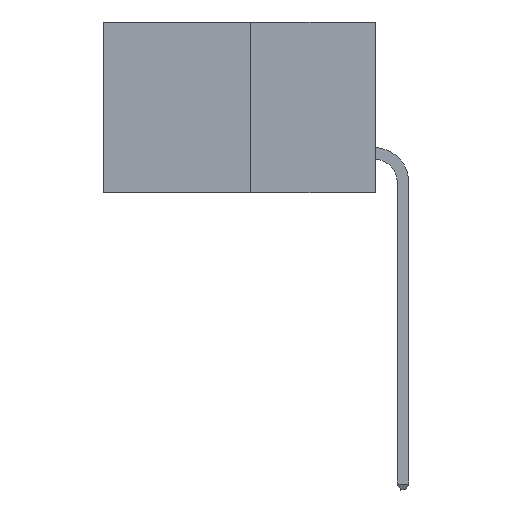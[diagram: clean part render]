
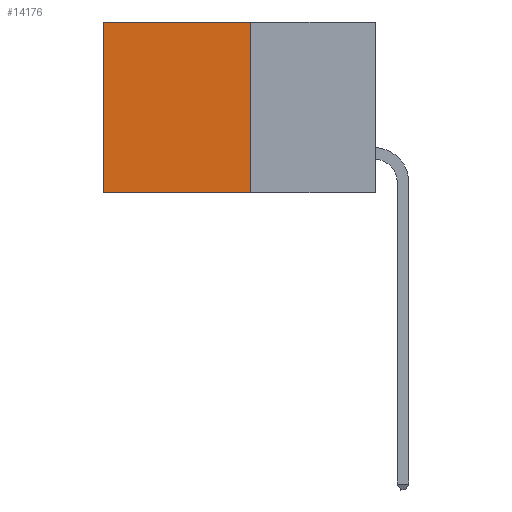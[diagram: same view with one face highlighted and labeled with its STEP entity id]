
A CAD part, left-side view. The second image highlights one B-rep face of the part: STEP entity #14176.
In plain terms, the highlighted planar face has unit normal (-1, 0, 0).
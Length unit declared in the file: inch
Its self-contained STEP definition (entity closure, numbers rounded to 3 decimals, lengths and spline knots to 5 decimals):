
#125 = CARTESIAN_POINT ( 'NONE',  ( 0.277, 0.27, -0.37 ) ) ;
#161 = VERTEX_POINT ( 'NONE', #10917 ) ;
#1393 = CARTESIAN_POINT ( 'NONE',  ( 0.277, 0.27, 0. ) ) ;
#2013 = CARTESIAN_POINT ( 'NONE',  ( 0.277, 0.27, -0.37 ) ) ;
#2103 = ORIENTED_EDGE ( 'NONE', *, *, #19118, .T. ) ;
#2330 = CARTESIAN_POINT ( 'NONE',  ( 0.277, 0.59, 0. ) ) ;
#2685 = VERTEX_POINT ( 'NONE', #1393 ) ;
#3333 = ORIENTED_EDGE ( 'NONE', *, *, #11061, .F. ) ;
#3602 = CARTESIAN_POINT ( 'NONE',  ( 0.277, 0.27, -0.37 ) ) ;
#3877 = VERTEX_POINT ( 'NONE', #3602 ) ;
#4051 = LINE ( 'NONE', #2013, #12838 ) ;
#4062 = CARTESIAN_POINT ( 'NONE',  ( 0.277, 0.27, -0.37 ) ) ;
#4515 = VECTOR ( 'NONE', #11590, 39.37008 ) ;
#4836 = LINE ( 'NONE', #14430, #19806 ) ;
#5049 = EDGE_CURVE ( 'NONE', #3877, #161, #4051, .T. ) ;
#5095 = LINE ( 'NONE', #125, #4515 ) ;
#5385 = LINE ( 'NONE', #15758, #20344 ) ;
#5937 = DIRECTION ( 'NONE',  ( 1., 0., 0. ) ) ;
#9110 = AXIS2_PLACEMENT_3D ( 'NONE', #4062, #5937, #19050 ) ;
#9390 = FACE_OUTER_BOUND ( 'NONE', #17616, .T. ) ;
#9659 = PLANE ( 'NONE',  #9110 ) ;
#10692 = DIRECTION ( 'NONE',  ( 0., 1., 0. ) ) ;
#10917 = CARTESIAN_POINT ( 'NONE',  ( 0.277, 0.59, -0.37 ) ) ;
#11061 = EDGE_CURVE ( 'NONE', #2685, #3877, #5095, .T. ) ;
#11224 = EDGE_CURVE ( 'NONE', #19503, #161, #5385, .T. ) ;
#11590 = DIRECTION ( 'NONE',  ( 0., 0., -1. ) ) ;
#12838 = VECTOR ( 'NONE', #22607, 39.37008 ) ;
#13923 = DIRECTION ( 'NONE',  ( 0., 0., -1. ) ) ;
#14176 = ADVANCED_FACE ( 'NONE', ( #9390 ), #9659, .F. ) ;
#14430 = CARTESIAN_POINT ( 'NONE',  ( 0.277, 0.27, 0. ) ) ;
#15758 = CARTESIAN_POINT ( 'NONE',  ( 0.277, 0.59, -0.37 ) ) ;
#17616 = EDGE_LOOP ( 'NONE', ( #21207, #24004, #3333, #2103 ) ) ;
#19050 = DIRECTION ( 'NONE',  ( 0., 0., -1. ) ) ;
#19118 = EDGE_CURVE ( 'NONE', #2685, #19503, #4836, .T. ) ;
#19503 = VERTEX_POINT ( 'NONE', #2330 ) ;
#19806 = VECTOR ( 'NONE', #10692, 39.37008 ) ;
#20344 = VECTOR ( 'NONE', #13923, 39.37008 ) ;
#21207 = ORIENTED_EDGE ( 'NONE', *, *, #11224, .T. ) ;
#22607 = DIRECTION ( 'NONE',  ( 0., 1., 0. ) ) ;
#24004 = ORIENTED_EDGE ( 'NONE', *, *, #5049, .F. ) ;
